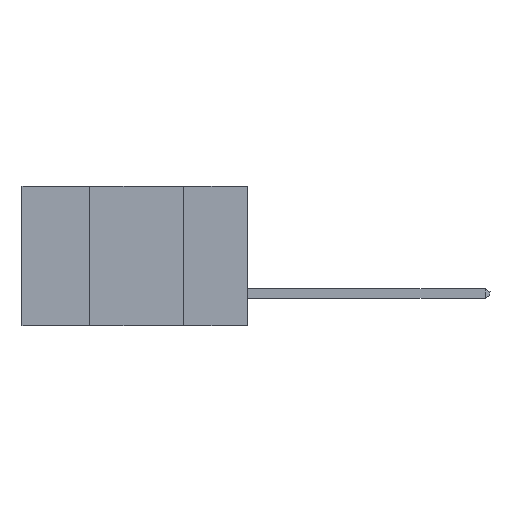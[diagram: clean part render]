
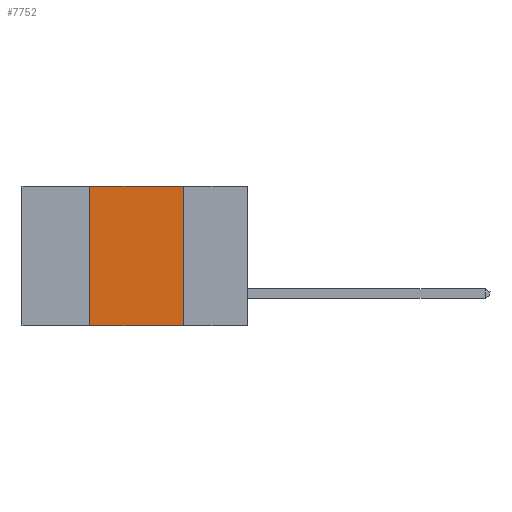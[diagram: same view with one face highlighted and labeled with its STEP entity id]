
A CAD part, left-side view. The second image highlights one B-rep face of the part: STEP entity #7752.
In plain terms, the highlighted planar face has unit normal (-1, 0, 0).
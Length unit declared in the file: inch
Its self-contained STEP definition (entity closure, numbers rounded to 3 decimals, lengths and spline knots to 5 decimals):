
#267 = VECTOR ( 'NONE', #3299, 39.37008 ) ;
#643 = LINE ( 'NONE', #4518, #1835 ) ;
#826 = ORIENTED_EDGE ( 'NONE', *, *, #6878, .F. ) ;
#1568 = LINE ( 'NONE', #5932, #6019 ) ;
#1835 = VECTOR ( 'NONE', #9162, 39.37008 ) ;
#2366 = VERTEX_POINT ( 'NONE', #9451 ) ;
#2573 = LINE ( 'NONE', #7186, #267 ) ;
#3299 = DIRECTION ( 'NONE',  ( 0., -1., 0. ) ) ;
#3345 = VERTEX_POINT ( 'NONE', #6842 ) ;
#3363 = EDGE_CURVE ( 'NONE', #7072, #2366, #643, .T. ) ;
#3381 = LINE ( 'NONE', #9024, #7295 ) ;
#3439 = ORIENTED_EDGE ( 'NONE', *, *, #6230, .F. ) ;
#3739 = VERTEX_POINT ( 'NONE', #8888 ) ;
#4518 = CARTESIAN_POINT ( 'NONE',  ( 0., 0.42, -0.37 ) ) ;
#4883 = DIRECTION ( 'NONE',  ( 1., 0., 0. ) ) ;
#4891 = DIRECTION ( 'NONE',  ( 0., -1., 0. ) ) ;
#5807 = EDGE_LOOP ( 'NONE', ( #826, #3439, #6231, #8930 ) ) ;
#5932 = CARTESIAN_POINT ( 'NONE',  ( 0., 0.17, -0.37 ) ) ;
#6019 = VECTOR ( 'NONE', #8293, 39.37008 ) ;
#6230 = EDGE_CURVE ( 'NONE', #2366, #3739, #3381, .T. ) ;
#6231 = ORIENTED_EDGE ( 'NONE', *, *, #3363, .F. ) ;
#6842 = CARTESIAN_POINT ( 'NONE',  ( 0., 0.17, -0.37 ) ) ;
#6878 = EDGE_CURVE ( 'NONE', #3739, #3345, #1568, .T. ) ;
#7072 = VERTEX_POINT ( 'NONE', #9849 ) ;
#7186 = CARTESIAN_POINT ( 'NONE',  ( 0., 0.6, -0.37 ) ) ;
#7295 = VECTOR ( 'NONE', #4891, 39.37008 ) ;
#7752 = ADVANCED_FACE ( 'NONE', ( #7930 ), #8811, .F. ) ;
#7930 = FACE_OUTER_BOUND ( 'NONE', #5807, .T. ) ;
#8151 = AXIS2_PLACEMENT_3D ( 'NONE', #9366, #4883, #9415 ) ;
#8293 = DIRECTION ( 'NONE',  ( 0., 0., -1. ) ) ;
#8773 = EDGE_CURVE ( 'NONE', #7072, #3345, #2573, .T. ) ;
#8811 = PLANE ( 'NONE',  #8151 ) ;
#8888 = CARTESIAN_POINT ( 'NONE',  ( 0., 0.17, 0. ) ) ;
#8930 = ORIENTED_EDGE ( 'NONE', *, *, #8773, .T. ) ;
#9024 = CARTESIAN_POINT ( 'NONE',  ( 0., 0.6, 0. ) ) ;
#9162 = DIRECTION ( 'NONE',  ( 0., 0., 1. ) ) ;
#9366 = CARTESIAN_POINT ( 'NONE',  ( 0., 0.6, 0. ) ) ;
#9415 = DIRECTION ( 'NONE',  ( 0., 0., -1. ) ) ;
#9451 = CARTESIAN_POINT ( 'NONE',  ( 0., 0.42, 0. ) ) ;
#9849 = CARTESIAN_POINT ( 'NONE',  ( 0., 0.42, -0.37 ) ) ;
